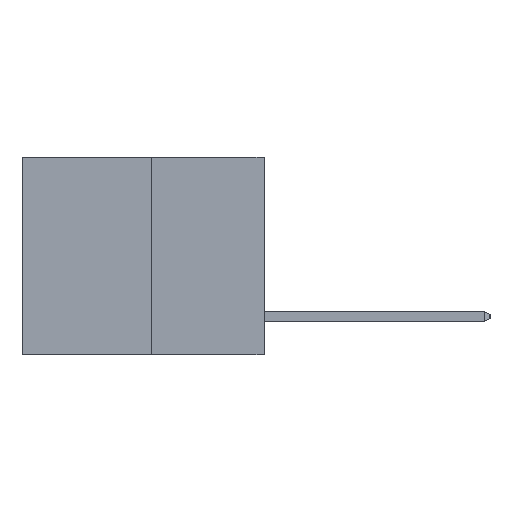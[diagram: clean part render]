
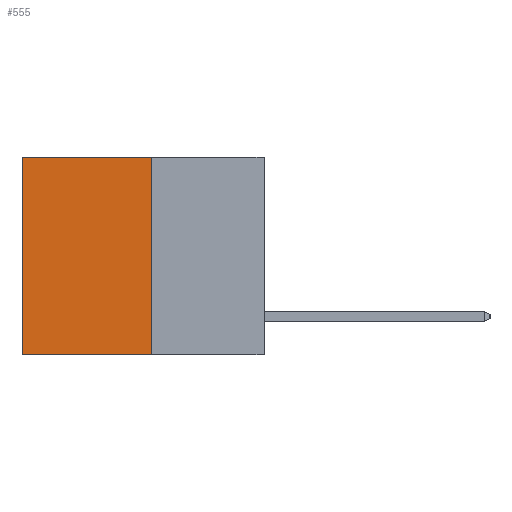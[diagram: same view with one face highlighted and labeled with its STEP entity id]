
A CAD part, left-side view. The second image highlights one B-rep face of the part: STEP entity #555.
In plain terms, the highlighted planar face has unit normal (-1, 0, 0).
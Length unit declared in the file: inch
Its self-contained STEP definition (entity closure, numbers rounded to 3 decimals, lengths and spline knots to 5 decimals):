
#555 = ADVANCED_FACE ( 'NONE', ( #17939 ), #27288, .F. ) ;
#1025 = ORIENTED_EDGE ( 'NONE', *, *, #6710, .T. ) ;
#1402 = EDGE_LOOP ( 'NONE', ( #9537, #7142, #3256, #1025 ) ) ;
#3247 = DIRECTION ( 'NONE',  ( 0., 0., -1. ) ) ;
#3256 = ORIENTED_EDGE ( 'NONE', *, *, #10207, .F. ) ;
#3289 = DIRECTION ( 'NONE',  ( 0., 0., -1. ) ) ;
#3343 = CARTESIAN_POINT ( 'NONE',  ( 0.3165, 0.28, -0.49 ) ) ;
#3851 = VERTEX_POINT ( 'NONE', #18711 ) ;
#4074 = LINE ( 'NONE', #14128, #10847 ) ;
#6710 = EDGE_CURVE ( 'NONE', #3851, #8887, #11989, .T. ) ;
#7097 = CARTESIAN_POINT ( 'NONE',  ( 0.3165, 0.28, -0.49 ) ) ;
#7142 = ORIENTED_EDGE ( 'NONE', *, *, #27056, .F. ) ;
#8333 = EDGE_CURVE ( 'NONE', #8887, #11067, #4074, .T. ) ;
#8887 = VERTEX_POINT ( 'NONE', #16179 ) ;
#9537 = ORIENTED_EDGE ( 'NONE', *, *, #8333, .T. ) ;
#10207 = EDGE_CURVE ( 'NONE', #3851, #25318, #15837, .T. ) ;
#10847 = VECTOR ( 'NONE', #3289, 39.37008 ) ;
#11067 = VERTEX_POINT ( 'NONE', #18380 ) ;
#11989 = LINE ( 'NONE', #27836, #26224 ) ;
#14128 = CARTESIAN_POINT ( 'NONE',  ( 0.3165, 0.6, -0.49 ) ) ;
#14839 = DIRECTION ( 'NONE',  ( 0., 1., 0. ) ) ;
#15188 = LINE ( 'NONE', #3343, #19586 ) ;
#15837 = LINE ( 'NONE', #21721, #26697 ) ;
#16179 = CARTESIAN_POINT ( 'NONE',  ( 0.3165, 0.6, 0. ) ) ;
#16377 = CARTESIAN_POINT ( 'NONE',  ( 0.3165, 0.28, -0.49 ) ) ;
#16557 = DIRECTION ( 'NONE',  ( 1., 0., 0. ) ) ;
#17939 = FACE_OUTER_BOUND ( 'NONE', #1402, .T. ) ;
#18380 = CARTESIAN_POINT ( 'NONE',  ( 0.3165, 0.6, -0.49 ) ) ;
#18538 = DIRECTION ( 'NONE',  ( 0., 1., 0. ) ) ;
#18711 = CARTESIAN_POINT ( 'NONE',  ( 0.3165, 0.28, 0. ) ) ;
#19586 = VECTOR ( 'NONE', #18538, 39.37008 ) ;
#21540 = AXIS2_PLACEMENT_3D ( 'NONE', #16377, #16557, #3247 ) ;
#21721 = CARTESIAN_POINT ( 'NONE',  ( 0.3165, 0.28, -0.49 ) ) ;
#23727 = DIRECTION ( 'NONE',  ( 0., 0., -1. ) ) ;
#25318 = VERTEX_POINT ( 'NONE', #7097 ) ;
#26224 = VECTOR ( 'NONE', #14839, 39.37008 ) ;
#26697 = VECTOR ( 'NONE', #23727, 39.37008 ) ;
#27056 = EDGE_CURVE ( 'NONE', #25318, #11067, #15188, .T. ) ;
#27288 = PLANE ( 'NONE',  #21540 ) ;
#27836 = CARTESIAN_POINT ( 'NONE',  ( 0.3165, 0.28, 0. ) ) ;
